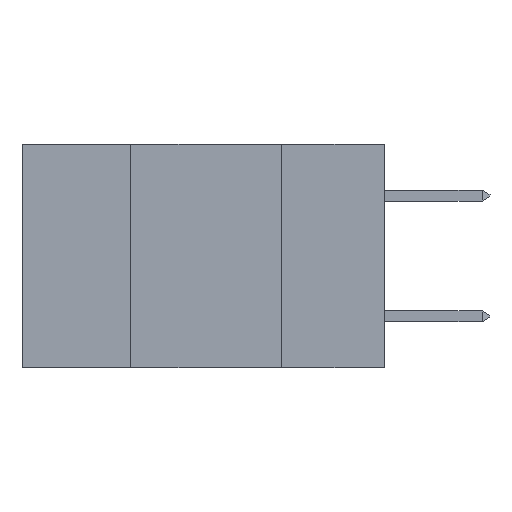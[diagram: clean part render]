
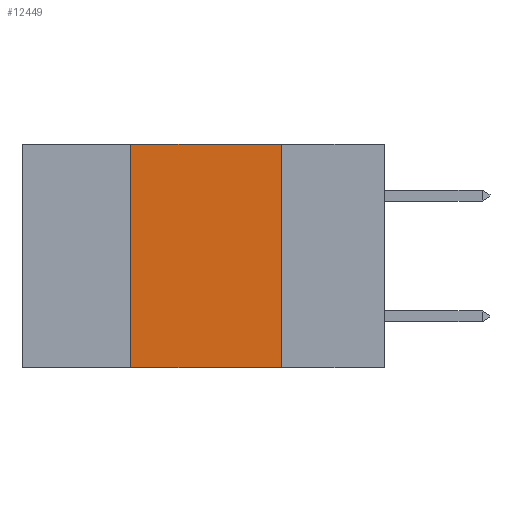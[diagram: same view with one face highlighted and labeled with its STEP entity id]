
A CAD part, left-side view. The second image highlights one B-rep face of the part: STEP entity #12449.
In plain terms, the highlighted planar face has unit normal (-1, 0, 0).
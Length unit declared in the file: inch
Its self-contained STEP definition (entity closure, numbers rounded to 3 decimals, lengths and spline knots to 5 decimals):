
#175 = CARTESIAN_POINT ( 'NONE',  ( 0., 0.6, 0. ) ) ;
#639 = CARTESIAN_POINT ( 'NONE',  ( 0., 0.6, 0. ) ) ;
#1008 = VERTEX_POINT ( 'NONE', #16507 ) ;
#2186 = VERTEX_POINT ( 'NONE', #6150 ) ;
#2227 = VERTEX_POINT ( 'NONE', #3511 ) ;
#2595 = DIRECTION ( 'NONE',  ( 0., 0., 1. ) ) ;
#3511 = CARTESIAN_POINT ( 'NONE',  ( 0., 0.42, 0. ) ) ;
#4287 = VECTOR ( 'NONE', #11735, 39.37008 ) ;
#4875 = EDGE_CURVE ( 'NONE', #1008, #2186, #5379, .T. ) ;
#5379 = LINE ( 'NONE', #10321, #4287 ) ;
#5510 = FACE_OUTER_BOUND ( 'NONE', #12417, .T. ) ;
#6150 = CARTESIAN_POINT ( 'NONE',  ( 0., 0.17, -0.37 ) ) ;
#6299 = VERTEX_POINT ( 'NONE', #15068 ) ;
#6341 = VECTOR ( 'NONE', #17437, 39.37008 ) ;
#6782 = LINE ( 'NONE', #639, #6341 ) ;
#7756 = CARTESIAN_POINT ( 'NONE',  ( 0., 0.6, -0.37 ) ) ;
#7769 = LINE ( 'NONE', #15216, #14808 ) ;
#8055 = AXIS2_PLACEMENT_3D ( 'NONE', #175, #11403, #15394 ) ;
#8186 = VECTOR ( 'NONE', #9150, 39.37008 ) ;
#8841 = ORIENTED_EDGE ( 'NONE', *, *, #10394, .T. ) ;
#9150 = DIRECTION ( 'NONE',  ( 0., -1., 0. ) ) ;
#10321 = CARTESIAN_POINT ( 'NONE',  ( 0., 0.17, 0. ) ) ;
#10394 = EDGE_CURVE ( 'NONE', #6299, #2186, #14583, .T. ) ;
#11209 = PLANE ( 'NONE',  #8055 ) ;
#11403 = DIRECTION ( 'NONE',  ( 1., 0., 0. ) ) ;
#11735 = DIRECTION ( 'NONE',  ( 0., 0., -1. ) ) ;
#12417 = EDGE_LOOP ( 'NONE', ( #17977, #14836, #16176, #8841 ) ) ;
#12449 = ADVANCED_FACE ( 'NONE', ( #5510 ), #11209, .F. ) ;
#14434 = EDGE_CURVE ( 'NONE', #2227, #1008, #6782, .T. ) ;
#14583 = LINE ( 'NONE', #7756, #8186 ) ;
#14808 = VECTOR ( 'NONE', #2595, 39.37008 ) ;
#14836 = ORIENTED_EDGE ( 'NONE', *, *, #14434, .F. ) ;
#15068 = CARTESIAN_POINT ( 'NONE',  ( 0., 0.42, -0.37 ) ) ;
#15216 = CARTESIAN_POINT ( 'NONE',  ( 0., 0.42, 0. ) ) ;
#15394 = DIRECTION ( 'NONE',  ( 0., 0., -1. ) ) ;
#16176 = ORIENTED_EDGE ( 'NONE', *, *, #16280, .F. ) ;
#16280 = EDGE_CURVE ( 'NONE', #6299, #2227, #7769, .T. ) ;
#16507 = CARTESIAN_POINT ( 'NONE',  ( 0., 0.17, 0. ) ) ;
#17437 = DIRECTION ( 'NONE',  ( 0., -1., 0. ) ) ;
#17977 = ORIENTED_EDGE ( 'NONE', *, *, #4875, .F. ) ;
